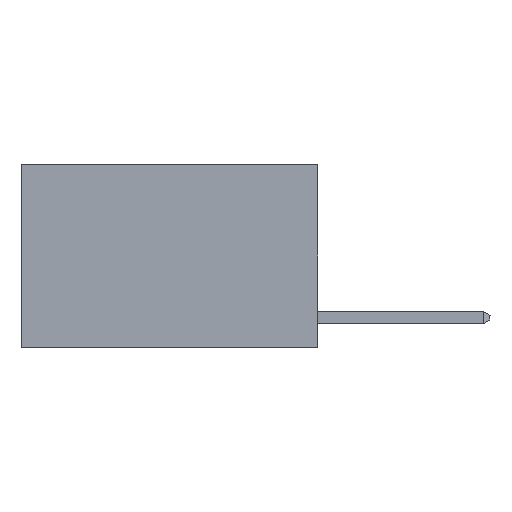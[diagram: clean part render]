
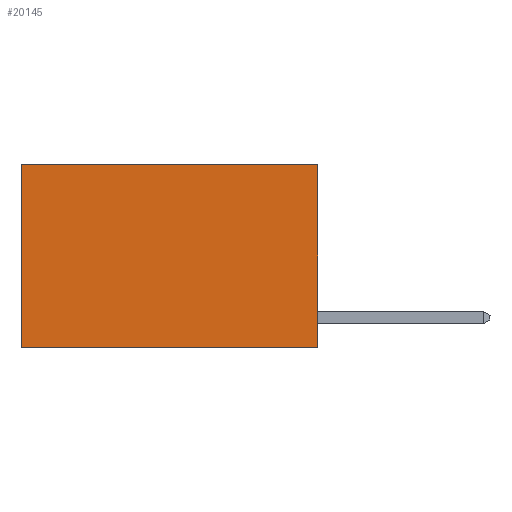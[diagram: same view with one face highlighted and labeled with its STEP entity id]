
A CAD part, left-side view. The second image highlights one B-rep face of the part: STEP entity #20145.
In plain terms, the highlighted planar face has unit normal (-1, 0, 0).
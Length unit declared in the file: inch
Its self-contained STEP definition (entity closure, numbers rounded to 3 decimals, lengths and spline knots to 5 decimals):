
#1438 = CARTESIAN_POINT ( 'NONE',  ( 0.2625, 0.6, 0. ) ) ;
#2153 = VECTOR ( 'NONE', #18669, 39.37008 ) ;
#2249 = EDGE_LOOP ( 'NONE', ( #12076, #13078, #12995, #14645 ) ) ;
#2672 = VERTEX_POINT ( 'NONE', #20009 ) ;
#3532 = VERTEX_POINT ( 'NONE', #6671 ) ;
#3746 = LINE ( 'NONE', #11131, #10530 ) ;
#3786 = VERTEX_POINT ( 'NONE', #11604 ) ;
#6671 = CARTESIAN_POINT ( 'NONE',  ( 0.2625, 0., -0.37 ) ) ;
#7597 = EDGE_CURVE ( 'NONE', #19089, #2672, #3746, .T. ) ;
#8340 = CARTESIAN_POINT ( 'NONE',  ( 0.2625, 0., 0. ) ) ;
#8485 = PLANE ( 'NONE',  #15529 ) ;
#10530 = VECTOR ( 'NONE', #11050, 39.37008 ) ;
#11050 = DIRECTION ( 'NONE',  ( 0., 1., 0. ) ) ;
#11131 = CARTESIAN_POINT ( 'NONE',  ( 0.2625, 0., 0. ) ) ;
#11175 = LINE ( 'NONE', #20253, #2153 ) ;
#11604 = CARTESIAN_POINT ( 'NONE',  ( 0.2625, 0.6, -0.37 ) ) ;
#11694 = DIRECTION ( 'NONE',  ( 0., 0., -1. ) ) ;
#12076 = ORIENTED_EDGE ( 'NONE', *, *, #14367, .T. ) ;
#12196 = DIRECTION ( 'NONE',  ( 0., 0., -1. ) ) ;
#12966 = LINE ( 'NONE', #1438, #19138 ) ;
#12995 = ORIENTED_EDGE ( 'NONE', *, *, #22079, .F. ) ;
#13078 = ORIENTED_EDGE ( 'NONE', *, *, #16750, .F. ) ;
#13834 = DIRECTION ( 'NONE',  ( 0., 0., -1. ) ) ;
#14367 = EDGE_CURVE ( 'NONE', #2672, #3786, #12966, .T. ) ;
#14645 = ORIENTED_EDGE ( 'NONE', *, *, #7597, .T. ) ;
#15529 = AXIS2_PLACEMENT_3D ( 'NONE', #8340, #17334, #13834 ) ;
#16109 = CARTESIAN_POINT ( 'NONE',  ( 0.2625, 0., 0. ) ) ;
#16750 = EDGE_CURVE ( 'NONE', #3532, #3786, #11175, .T. ) ;
#16957 = FACE_OUTER_BOUND ( 'NONE', #2249, .T. ) ;
#17154 = CARTESIAN_POINT ( 'NONE',  ( 0.2625, 0., 0. ) ) ;
#17334 = DIRECTION ( 'NONE',  ( 1., 0., 0. ) ) ;
#18669 = DIRECTION ( 'NONE',  ( 0., 1., 0. ) ) ;
#19089 = VERTEX_POINT ( 'NONE', #16109 ) ;
#19138 = VECTOR ( 'NONE', #11694, 39.37008 ) ;
#20009 = CARTESIAN_POINT ( 'NONE',  ( 0.2625, 0.6, 0. ) ) ;
#20145 = ADVANCED_FACE ( 'NONE', ( #16957 ), #8485, .F. ) ;
#20253 = CARTESIAN_POINT ( 'NONE',  ( 0.2625, 0., -0.37 ) ) ;
#20882 = LINE ( 'NONE', #17154, #22303 ) ;
#22079 = EDGE_CURVE ( 'NONE', #19089, #3532, #20882, .T. ) ;
#22303 = VECTOR ( 'NONE', #12196, 39.37008 ) ;
